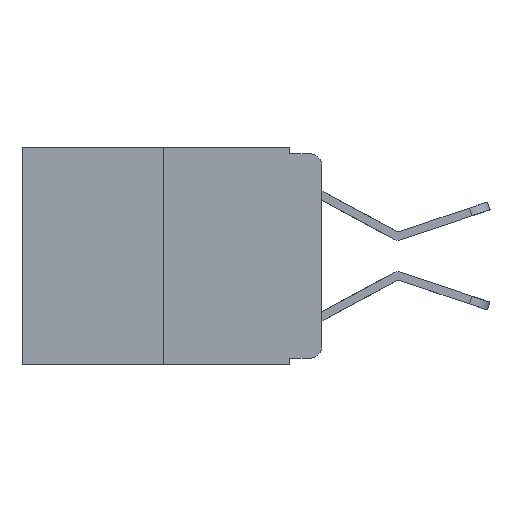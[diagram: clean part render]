
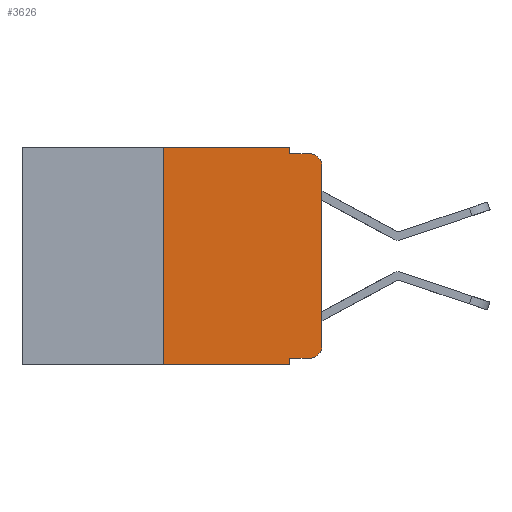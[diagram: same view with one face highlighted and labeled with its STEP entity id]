
A CAD part, left-side view. The second image highlights one B-rep face of the part: STEP entity #3626.
In plain terms, the highlighted planar face has unit normal (-1, 0, 0).
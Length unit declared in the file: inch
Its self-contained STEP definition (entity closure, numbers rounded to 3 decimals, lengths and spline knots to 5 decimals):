
#256 = DIRECTION ( 'NONE',  ( -1., 0., 0. ) ) ;
#342 = EDGE_CURVE ( 'NONE', #11550, #18294, #11319, .T. ) ;
#554 = CARTESIAN_POINT ( 'NONE',  ( 0., 0.02, -0.313 ) ) ;
#597 = CARTESIAN_POINT ( 'NONE',  ( 0., 0.051, -0.01 ) ) ;
#622 = VECTOR ( 'NONE', #7263, 39.37008 ) ;
#630 = VECTOR ( 'NONE', #8055, 39.37008 ) ;
#811 = VERTEX_POINT ( 'NONE', #14183 ) ;
#1166 = LINE ( 'NONE', #597, #622 ) ;
#1367 = CIRCLE ( 'NONE', #12033, 0.02 ) ;
#1477 = EDGE_CURVE ( 'NONE', #18294, #5440, #1166, .T. ) ;
#1709 = EDGE_LOOP ( 'NONE', ( #6908, #4921, #17981, #9923, #11204, #4078, #3096, #19203, #19742, #6195 ) ) ;
#1810 = VERTEX_POINT ( 'NONE', #9708 ) ;
#2274 = DIRECTION ( 'NONE',  ( 0., 0., -1. ) ) ;
#2363 = VERTEX_POINT ( 'NONE', #2864 ) ;
#2616 = EDGE_CURVE ( 'NONE', #6462, #5440, #1367, .T. ) ;
#2663 = VECTOR ( 'NONE', #10102, 39.37008 ) ;
#2864 = CARTESIAN_POINT ( 'NONE',  ( 0., 0.051, -0.343 ) ) ;
#2916 = VECTOR ( 'NONE', #9775, 39.37008 ) ;
#3096 = ORIENTED_EDGE ( 'NONE', *, *, #16350, .T. ) ;
#3626 = ADVANCED_FACE ( 'NONE', ( #20317 ), #14182, .F. ) ;
#3728 = EDGE_CURVE ( 'NONE', #6219, #6462, #18835, .T. ) ;
#4078 = ORIENTED_EDGE ( 'NONE', *, *, #20325, .F. ) ;
#4096 = CARTESIAN_POINT ( 'NONE',  ( 0., 0.051, -0.01 ) ) ;
#4491 = CARTESIAN_POINT ( 'NONE',  ( 0., 0., -0.03 ) ) ;
#4921 = ORIENTED_EDGE ( 'NONE', *, *, #2616, .T. ) ;
#5440 = VERTEX_POINT ( 'NONE', #19586 ) ;
#5470 = DIRECTION ( 'NONE',  ( 0., -1., 0. ) ) ;
#6073 = AXIS2_PLACEMENT_3D ( 'NONE', #15793, #10920, #17383 ) ;
#6195 = ORIENTED_EDGE ( 'NONE', *, *, #17136, .T. ) ;
#6219 = VERTEX_POINT ( 'NONE', #13582 ) ;
#6462 = VERTEX_POINT ( 'NONE', #4491 ) ;
#6908 = ORIENTED_EDGE ( 'NONE', *, *, #3728, .T. ) ;
#7263 = DIRECTION ( 'NONE',  ( 0., -1., 0. ) ) ;
#7616 = LINE ( 'NONE', #13257, #14668 ) ;
#8055 = DIRECTION ( 'NONE',  ( 0., 0., -1. ) ) ;
#9037 = CARTESIAN_POINT ( 'NONE',  ( 0., 0.051, 0. ) ) ;
#9079 = VECTOR ( 'NONE', #14317, 39.37008 ) ;
#9339 = EDGE_CURVE ( 'NONE', #19363, #11550, #10038, .T. ) ;
#9708 = CARTESIAN_POINT ( 'NONE',  ( 0., 0.02, -0.333 ) ) ;
#9775 = DIRECTION ( 'NONE',  ( 0., -1., 0. ) ) ;
#9776 = VECTOR ( 'NONE', #16348, 39.37008 ) ;
#9923 = ORIENTED_EDGE ( 'NONE', *, *, #342, .F. ) ;
#10038 = LINE ( 'NONE', #17777, #2916 ) ;
#10101 = CARTESIAN_POINT ( 'NONE',  ( 0., 0.02, -0.03 ) ) ;
#10102 = DIRECTION ( 'NONE',  ( 0., 0., -1. ) ) ;
#10920 = DIRECTION ( 'NONE',  ( 1., 0., 0. ) ) ;
#11002 = AXIS2_PLACEMENT_3D ( 'NONE', #554, #12040, #2274 ) ;
#11011 = VERTEX_POINT ( 'NONE', #11137 ) ;
#11137 = CARTESIAN_POINT ( 'NONE',  ( 0., 0.051, -0.333 ) ) ;
#11204 = ORIENTED_EDGE ( 'NONE', *, *, #9339, .F. ) ;
#11319 = LINE ( 'NONE', #9037, #2663 ) ;
#11550 = VERTEX_POINT ( 'NONE', #15693 ) ;
#11586 = CARTESIAN_POINT ( 'NONE',  ( 0., 0.25, 0. ) ) ;
#11737 = DIRECTION ( 'NONE',  ( 0., 0., -1. ) ) ;
#12033 = AXIS2_PLACEMENT_3D ( 'NONE', #10101, #256, #11737 ) ;
#12040 = DIRECTION ( 'NONE',  ( -1., 0., 0. ) ) ;
#12951 = CARTESIAN_POINT ( 'NONE',  ( 0., 0.051, 0. ) ) ;
#13087 = VECTOR ( 'NONE', #5470, 39.37008 ) ;
#13195 = DIRECTION ( 'NONE',  ( 0., -1., 0. ) ) ;
#13257 = CARTESIAN_POINT ( 'NONE',  ( 0., 0.473, -0.343 ) ) ;
#13582 = CARTESIAN_POINT ( 'NONE',  ( 0., 0., -0.313 ) ) ;
#13686 = LINE ( 'NONE', #12951, #630 ) ;
#13898 = LINE ( 'NONE', #19120, #9079 ) ;
#14099 = LINE ( 'NONE', #18289, #13087 ) ;
#14182 = PLANE ( 'NONE',  #6073 ) ;
#14183 = CARTESIAN_POINT ( 'NONE',  ( 0., 0.25, -0.343 ) ) ;
#14317 = DIRECTION ( 'NONE',  ( 0., 0., 1. ) ) ;
#14668 = VECTOR ( 'NONE', #13195, 39.37008 ) ;
#14727 = CARTESIAN_POINT ( 'NONE',  ( 0., 0., 0. ) ) ;
#15693 = CARTESIAN_POINT ( 'NONE',  ( 0., 0.051, 0. ) ) ;
#15793 = CARTESIAN_POINT ( 'NONE',  ( 0., 0.473, 0. ) ) ;
#16348 = DIRECTION ( 'NONE',  ( 0., 0., 1. ) ) ;
#16350 = EDGE_CURVE ( 'NONE', #811, #2363, #7616, .T. ) ;
#17136 = EDGE_CURVE ( 'NONE', #1810, #6219, #17632, .T. ) ;
#17383 = DIRECTION ( 'NONE',  ( 0., 0., -1. ) ) ;
#17632 = CIRCLE ( 'NONE', #11002, 0.02 ) ;
#17777 = CARTESIAN_POINT ( 'NONE',  ( 0., 0.473, 0. ) ) ;
#17981 = ORIENTED_EDGE ( 'NONE', *, *, #1477, .F. ) ;
#18191 = EDGE_CURVE ( 'NONE', #11011, #1810, #14099, .T. ) ;
#18289 = CARTESIAN_POINT ( 'NONE',  ( 0., 0.051, -0.333 ) ) ;
#18294 = VERTEX_POINT ( 'NONE', #4096 ) ;
#18835 = LINE ( 'NONE', #14727, #9776 ) ;
#19120 = CARTESIAN_POINT ( 'NONE',  ( 0., 0.25, 0. ) ) ;
#19203 = ORIENTED_EDGE ( 'NONE', *, *, #19251, .F. ) ;
#19251 = EDGE_CURVE ( 'NONE', #11011, #2363, #13686, .T. ) ;
#19363 = VERTEX_POINT ( 'NONE', #11586 ) ;
#19586 = CARTESIAN_POINT ( 'NONE',  ( 0., 0.02, -0.01 ) ) ;
#19742 = ORIENTED_EDGE ( 'NONE', *, *, #18191, .T. ) ;
#20317 = FACE_OUTER_BOUND ( 'NONE', #1709, .T. ) ;
#20325 = EDGE_CURVE ( 'NONE', #811, #19363, #13898, .T. ) ;
